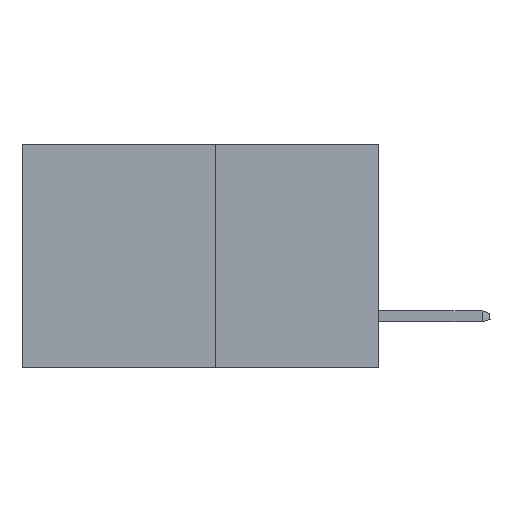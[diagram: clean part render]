
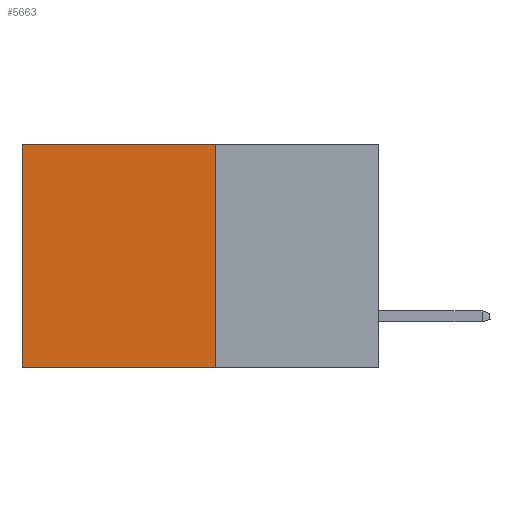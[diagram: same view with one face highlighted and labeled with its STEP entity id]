
A CAD part, left-side view. The second image highlights one B-rep face of the part: STEP entity #5663.
In plain terms, the highlighted planar face has unit normal (-1, 0, 0).
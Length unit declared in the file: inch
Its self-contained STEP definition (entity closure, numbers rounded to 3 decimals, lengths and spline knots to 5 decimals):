
#235 = VECTOR ( 'NONE', #1635, 39.37008 ) ;
#315 = EDGE_CURVE ( 'NONE', #9654, #10417, #3099, .T. ) ;
#606 = CARTESIAN_POINT ( 'NONE',  ( 0.277, 0.59, -0.37 ) ) ;
#1094 = DIRECTION ( 'NONE',  ( 0., 1., 0. ) ) ;
#1295 = ORIENTED_EDGE ( 'NONE', *, *, #3169, .F. ) ;
#1635 = DIRECTION ( 'NONE',  ( 0., 1., 0. ) ) ;
#1831 = CARTESIAN_POINT ( 'NONE',  ( 0.277, 0.27, -0.37 ) ) ;
#1937 = PLANE ( 'NONE',  #2956 ) ;
#1965 = VECTOR ( 'NONE', #8292, 39.37008 ) ;
#2956 = AXIS2_PLACEMENT_3D ( 'NONE', #12017, #3192, #4334 ) ;
#2984 = ORIENTED_EDGE ( 'NONE', *, *, #10377, .T. ) ;
#3099 = LINE ( 'NONE', #10471, #235 ) ;
#3141 = ORIENTED_EDGE ( 'NONE', *, *, #315, .T. ) ;
#3169 = EDGE_CURVE ( 'NONE', #4650, #12008, #5720, .T. ) ;
#3192 = DIRECTION ( 'NONE',  ( 1., 0., 0. ) ) ;
#3757 = CARTESIAN_POINT ( 'NONE',  ( 0.277, 0.59, -0.37 ) ) ;
#4334 = DIRECTION ( 'NONE',  ( 0., 0., -1. ) ) ;
#4423 = EDGE_CURVE ( 'NONE', #9654, #4650, #6697, .T. ) ;
#4650 = VERTEX_POINT ( 'NONE', #7997 ) ;
#4785 = FACE_OUTER_BOUND ( 'NONE', #10240, .T. ) ;
#5106 = CARTESIAN_POINT ( 'NONE',  ( 0.277, 0.27, 0. ) ) ;
#5422 = VECTOR ( 'NONE', #1094, 39.37008 ) ;
#5663 = ADVANCED_FACE ( 'NONE', ( #4785 ), #1937, .F. ) ;
#5720 = LINE ( 'NONE', #1831, #5422 ) ;
#6579 = CARTESIAN_POINT ( 'NONE',  ( 0.277, 0.59, 0. ) ) ;
#6697 = LINE ( 'NONE', #9236, #1965 ) ;
#7452 = ORIENTED_EDGE ( 'NONE', *, *, #4423, .F. ) ;
#7997 = CARTESIAN_POINT ( 'NONE',  ( 0.277, 0.27, -0.37 ) ) ;
#8287 = VECTOR ( 'NONE', #10262, 39.37008 ) ;
#8292 = DIRECTION ( 'NONE',  ( 0., 0., -1. ) ) ;
#9236 = CARTESIAN_POINT ( 'NONE',  ( 0.277, 0.27, -0.37 ) ) ;
#9654 = VERTEX_POINT ( 'NONE', #5106 ) ;
#10240 = EDGE_LOOP ( 'NONE', ( #2984, #1295, #7452, #3141 ) ) ;
#10262 = DIRECTION ( 'NONE',  ( 0., 0., -1. ) ) ;
#10377 = EDGE_CURVE ( 'NONE', #10417, #12008, #10458, .T. ) ;
#10417 = VERTEX_POINT ( 'NONE', #6579 ) ;
#10458 = LINE ( 'NONE', #3757, #8287 ) ;
#10471 = CARTESIAN_POINT ( 'NONE',  ( 0.277, 0.27, 0. ) ) ;
#12008 = VERTEX_POINT ( 'NONE', #606 ) ;
#12017 = CARTESIAN_POINT ( 'NONE',  ( 0.277, 0.27, -0.37 ) ) ;
